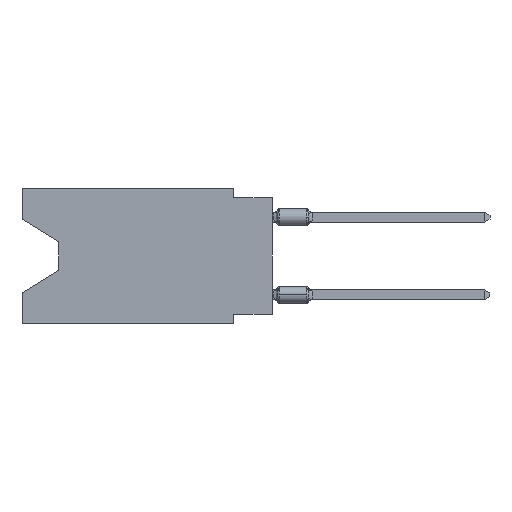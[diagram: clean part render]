
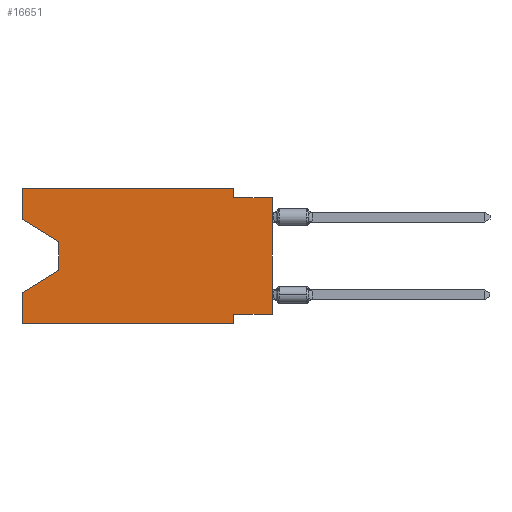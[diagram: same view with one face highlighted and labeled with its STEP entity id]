
A CAD part, left-side view. The second image highlights one B-rep face of the part: STEP entity #16651.
In plain terms, the highlighted planar face has unit normal (-1, 0, 0).
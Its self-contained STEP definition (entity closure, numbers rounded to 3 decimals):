
#100 = VECTOR ( 'NONE', #18810, 1000. ) ;
#541 = EDGE_CURVE ( 'NONE', #5117, #14129, #19291, .T. ) ;
#555 = CARTESIAN_POINT ( 'NONE',  ( 0., 16.383, -8.89 ) ) ;
#1147 = CARTESIAN_POINT ( 'NONE',  ( 0., 2.54, -0.635 ) ) ;
#1186 = VERTEX_POINT ( 'NONE', #555 ) ;
#1283 = DIRECTION ( 'NONE',  ( 0., 0., -1. ) ) ;
#1591 = DIRECTION ( 'NONE',  ( 0., -1., 0. ) ) ;
#2114 = VECTOR ( 'NONE', #9696, 1000. ) ;
#2331 = EDGE_CURVE ( 'NONE', #12142, #18245, #22241, .T. ) ;
#2546 = CARTESIAN_POINT ( 'NONE',  ( 0., 16.383, 0. ) ) ;
#2621 = VECTOR ( 'NONE', #9508, 1000. ) ;
#2943 = CARTESIAN_POINT ( 'NONE',  ( 0., 2.54, 0. ) ) ;
#3169 = ORIENTED_EDGE ( 'NONE', *, *, #2331, .F. ) ;
#3403 = VERTEX_POINT ( 'NONE', #4511 ) ;
#3505 = CARTESIAN_POINT ( 'NONE',  ( 0., 13.97, -5.385 ) ) ;
#3741 = CARTESIAN_POINT ( 'NONE',  ( 0., 2.54, -8.89 ) ) ;
#3748 = ORIENTED_EDGE ( 'NONE', *, *, #7061, .T. ) ;
#3792 = EDGE_CURVE ( 'NONE', #6696, #5117, #11698, .T. ) ;
#3999 = DIRECTION ( 'NONE',  ( 1., 0., 0. ) ) ;
#4247 = VERTEX_POINT ( 'NONE', #1147 ) ;
#4511 = CARTESIAN_POINT ( 'NONE',  ( 0., 16.383, 0. ) ) ;
#4870 = LINE ( 'NONE', #8388, #16554 ) ;
#5117 = VERTEX_POINT ( 'NONE', #13721 ) ;
#5355 = LINE ( 'NONE', #8875, #15312 ) ;
#5357 = EDGE_CURVE ( 'NONE', #1186, #14129, #19791, .T. ) ;
#6084 = LINE ( 'NONE', #7849, #12174 ) ;
#6300 = DIRECTION ( 'NONE',  ( 0., -1., 0. ) ) ;
#6458 = VERTEX_POINT ( 'NONE', #6936 ) ;
#6677 = DIRECTION ( 'NONE',  ( 0., 0., -1. ) ) ;
#6696 = VERTEX_POINT ( 'NONE', #20487 ) ;
#6936 = CARTESIAN_POINT ( 'NONE',  ( 0., 2.54, 0. ) ) ;
#7061 = EDGE_CURVE ( 'NONE', #1186, #18245, #6084, .T. ) ;
#7114 = VECTOR ( 'NONE', #9971, 1000. ) ;
#7236 = DIRECTION ( 'NONE',  ( 0., -0.855, -0.519 ) ) ;
#7389 = ORIENTED_EDGE ( 'NONE', *, *, #18648, .T. ) ;
#7458 = EDGE_CURVE ( 'NONE', #21417, #3403, #21851, .T. ) ;
#7674 = ORIENTED_EDGE ( 'NONE', *, *, #3792, .T. ) ;
#7678 = CARTESIAN_POINT ( 'NONE',  ( 0., 16.383, -2.038 ) ) ;
#7849 = CARTESIAN_POINT ( 'NONE',  ( 0., 16.383, -8.89 ) ) ;
#8062 = LINE ( 'NONE', #22547, #9787 ) ;
#8388 = CARTESIAN_POINT ( 'NONE',  ( 0., 0., -0.635 ) ) ;
#8875 = CARTESIAN_POINT ( 'NONE',  ( 0., 16.383, -2.038 ) ) ;
#9151 = FACE_OUTER_BOUND ( 'NONE', #22139, .T. ) ;
#9177 = CARTESIAN_POINT ( 'NONE',  ( 0., 2.54, -8.255 ) ) ;
#9508 = DIRECTION ( 'NONE',  ( 0., 0., 1. ) ) ;
#9514 = AXIS2_PLACEMENT_3D ( 'NONE', #20023, #3999, #17066 ) ;
#9696 = DIRECTION ( 'NONE',  ( 0., 0., 1. ) ) ;
#9787 = VECTOR ( 'NONE', #6300, 1000. ) ;
#9873 = ORIENTED_EDGE ( 'NONE', *, *, #11207, .F. ) ;
#9971 = DIRECTION ( 'NONE',  ( 0., 0., -1. ) ) ;
#10143 = CARTESIAN_POINT ( 'NONE',  ( 0., 0., -0.635 ) ) ;
#10286 = CARTESIAN_POINT ( 'NONE',  ( 0., 13.97, -3.505 ) ) ;
#10306 = ORIENTED_EDGE ( 'NONE', *, *, #21212, .F. ) ;
#11117 = EDGE_CURVE ( 'NONE', #21417, #6696, #5355, .T. ) ;
#11207 = EDGE_CURVE ( 'NONE', #6458, #4247, #22595, .T. ) ;
#11337 = DIRECTION ( 'NONE',  ( 0., -1., 0. ) ) ;
#11559 = ORIENTED_EDGE ( 'NONE', *, *, #22275, .F. ) ;
#11698 = LINE ( 'NONE', #10286, #14950 ) ;
#12142 = VERTEX_POINT ( 'NONE', #9177 ) ;
#12174 = VECTOR ( 'NONE', #11337, 1000. ) ;
#13495 = ORIENTED_EDGE ( 'NONE', *, *, #5357, .F. ) ;
#13695 = CARTESIAN_POINT ( 'NONE',  ( 0., 2.54, -8.89 ) ) ;
#13721 = CARTESIAN_POINT ( 'NONE',  ( 0., 13.97, -5.385 ) ) ;
#13988 = ORIENTED_EDGE ( 'NONE', *, *, #11117, .T. ) ;
#14072 = ORIENTED_EDGE ( 'NONE', *, *, #14478, .F. ) ;
#14129 = VERTEX_POINT ( 'NONE', #22816 ) ;
#14157 = DIRECTION ( 'NONE',  ( 0., 0.855, -0.519 ) ) ;
#14478 = EDGE_CURVE ( 'NONE', #14897, #12142, #17404, .T. ) ;
#14645 = PLANE ( 'NONE',  #9514 ) ;
#14897 = VERTEX_POINT ( 'NONE', #17256 ) ;
#14950 = VECTOR ( 'NONE', #6677, 1000. ) ;
#15312 = VECTOR ( 'NONE', #7236, 1000. ) ;
#15505 = CARTESIAN_POINT ( 'NONE',  ( 0., 0., 0. ) ) ;
#15620 = LINE ( 'NONE', #15505, #19589 ) ;
#15647 = ORIENTED_EDGE ( 'NONE', *, *, #7458, .F. ) ;
#16554 = VECTOR ( 'NONE', #1591, 1000. ) ;
#16651 = ADVANCED_FACE ( 'NONE', ( #9151 ), #14645, .F. ) ;
#16770 = VECTOR ( 'NONE', #1283, 1000. ) ;
#17066 = DIRECTION ( 'NONE',  ( 0., 0., -1. ) ) ;
#17256 = CARTESIAN_POINT ( 'NONE',  ( 0., 0., -8.255 ) ) ;
#17404 = LINE ( 'NONE', #20574, #100 ) ;
#18245 = VERTEX_POINT ( 'NONE', #3741 ) ;
#18263 = CARTESIAN_POINT ( 'NONE',  ( 0., 16.383, 0. ) ) ;
#18563 = VECTOR ( 'NONE', #14157, 1000. ) ;
#18648 = EDGE_CURVE ( 'NONE', #14897, #22419, #15620, .T. ) ;
#18810 = DIRECTION ( 'NONE',  ( 0., 1., 0. ) ) ;
#19240 = ORIENTED_EDGE ( 'NONE', *, *, #541, .T. ) ;
#19291 = LINE ( 'NONE', #3505, #18563 ) ;
#19589 = VECTOR ( 'NONE', #20539, 1000. ) ;
#19791 = LINE ( 'NONE', #18263, #2621 ) ;
#20023 = CARTESIAN_POINT ( 'NONE',  ( 0., 16.383, 0. ) ) ;
#20487 = CARTESIAN_POINT ( 'NONE',  ( 0., 13.97, -3.505 ) ) ;
#20539 = DIRECTION ( 'NONE',  ( 0., 0., 1. ) ) ;
#20574 = CARTESIAN_POINT ( 'NONE',  ( 0., 0., -8.255 ) ) ;
#21212 = EDGE_CURVE ( 'NONE', #4247, #22419, #4870, .T. ) ;
#21417 = VERTEX_POINT ( 'NONE', #7678 ) ;
#21851 = LINE ( 'NONE', #2546, #2114 ) ;
#22139 = EDGE_LOOP ( 'NONE', ( #13988, #7674, #19240, #13495, #3748, #3169, #14072, #7389, #10306, #9873, #11559, #15647 ) ) ;
#22241 = LINE ( 'NONE', #13695, #16770 ) ;
#22275 = EDGE_CURVE ( 'NONE', #3403, #6458, #8062, .T. ) ;
#22419 = VERTEX_POINT ( 'NONE', #10143 ) ;
#22547 = CARTESIAN_POINT ( 'NONE',  ( 0., 16.383, 0. ) ) ;
#22595 = LINE ( 'NONE', #2943, #7114 ) ;
#22816 = CARTESIAN_POINT ( 'NONE',  ( 0., 16.383, -6.852 ) ) ;
